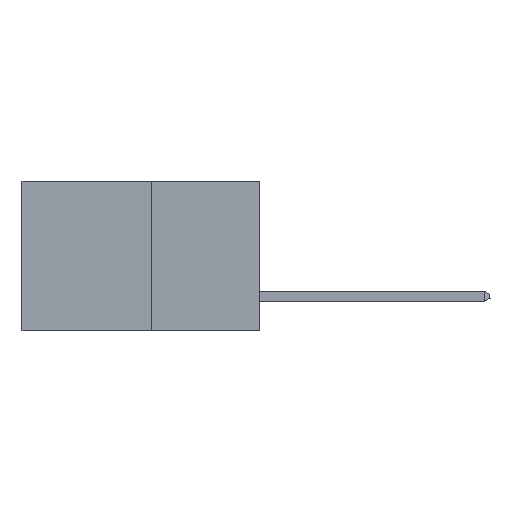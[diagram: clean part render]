
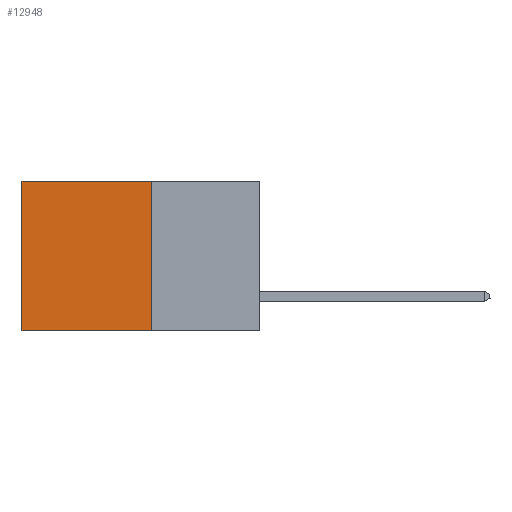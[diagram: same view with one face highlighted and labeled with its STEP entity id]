
A CAD part, left-side view. The second image highlights one B-rep face of the part: STEP entity #12948.
In plain terms, the highlighted planar face has unit normal (-1, 0, 0).
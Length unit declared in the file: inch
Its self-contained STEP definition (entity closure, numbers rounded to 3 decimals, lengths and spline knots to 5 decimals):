
#114 = DIRECTION ( 'NONE',  ( 0., 1., 0. ) ) ;
#1219 = EDGE_LOOP ( 'NONE', ( #1403, #1613, #16637, #11999 ) ) ;
#1360 = FACE_OUTER_BOUND ( 'NONE', #1219, .T. ) ;
#1403 = ORIENTED_EDGE ( 'NONE', *, *, #3761, .T. ) ;
#1613 = ORIENTED_EDGE ( 'NONE', *, *, #13455, .F. ) ;
#3406 = DIRECTION ( 'NONE',  ( 0., 0., -1. ) ) ;
#3761 = EDGE_CURVE ( 'NONE', #16917, #14121, #12735, .T. ) ;
#4092 = VECTOR ( 'NONE', #14106, 39.37008 ) ;
#5448 = DIRECTION ( 'NONE',  ( 0., 0., -1. ) ) ;
#5680 = VECTOR ( 'NONE', #5448, 39.37008 ) ;
#6745 = VERTEX_POINT ( 'NONE', #16131 ) ;
#6770 = CARTESIAN_POINT ( 'NONE',  ( 0.277, 0.59, -0.37 ) ) ;
#8571 = DIRECTION ( 'NONE',  ( 0., 0., -1. ) ) ;
#8753 = CARTESIAN_POINT ( 'NONE',  ( 0.277, 0.27, -0.37 ) ) ;
#10000 = LINE ( 'NONE', #8753, #16495 ) ;
#10384 = VECTOR ( 'NONE', #114, 39.37008 ) ;
#10956 = LINE ( 'NONE', #12775, #4092 ) ;
#11126 = VERTEX_POINT ( 'NONE', #16522 ) ;
#11999 = ORIENTED_EDGE ( 'NONE', *, *, #14995, .T. ) ;
#12079 = CARTESIAN_POINT ( 'NONE',  ( 0.277, 0.59, -0.37 ) ) ;
#12528 = AXIS2_PLACEMENT_3D ( 'NONE', #13831, #16378, #8571 ) ;
#12735 = LINE ( 'NONE', #12079, #5680 ) ;
#12775 = CARTESIAN_POINT ( 'NONE',  ( 0.277, 0.27, 0. ) ) ;
#12948 = ADVANCED_FACE ( 'NONE', ( #1360 ), #15125, .F. ) ;
#12996 = CARTESIAN_POINT ( 'NONE',  ( 0.277, 0.59, 0. ) ) ;
#13056 = EDGE_CURVE ( 'NONE', #11126, #6745, #10000, .T. ) ;
#13455 = EDGE_CURVE ( 'NONE', #6745, #14121, #16856, .T. ) ;
#13524 = CARTESIAN_POINT ( 'NONE',  ( 0.277, 0.27, -0.37 ) ) ;
#13831 = CARTESIAN_POINT ( 'NONE',  ( 0.277, 0.27, -0.37 ) ) ;
#14106 = DIRECTION ( 'NONE',  ( 0., 1., 0. ) ) ;
#14121 = VERTEX_POINT ( 'NONE', #6770 ) ;
#14995 = EDGE_CURVE ( 'NONE', #11126, #16917, #10956, .T. ) ;
#15125 = PLANE ( 'NONE',  #12528 ) ;
#16131 = CARTESIAN_POINT ( 'NONE',  ( 0.277, 0.27, -0.37 ) ) ;
#16378 = DIRECTION ( 'NONE',  ( 1., 0., 0. ) ) ;
#16495 = VECTOR ( 'NONE', #3406, 39.37008 ) ;
#16522 = CARTESIAN_POINT ( 'NONE',  ( 0.277, 0.27, 0. ) ) ;
#16637 = ORIENTED_EDGE ( 'NONE', *, *, #13056, .F. ) ;
#16856 = LINE ( 'NONE', #13524, #10384 ) ;
#16917 = VERTEX_POINT ( 'NONE', #12996 ) ;
